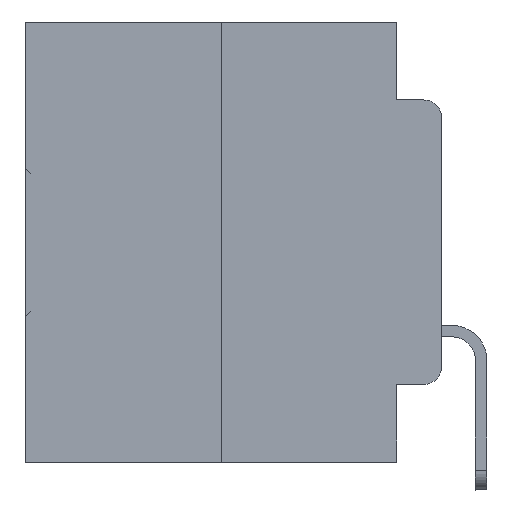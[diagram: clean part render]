
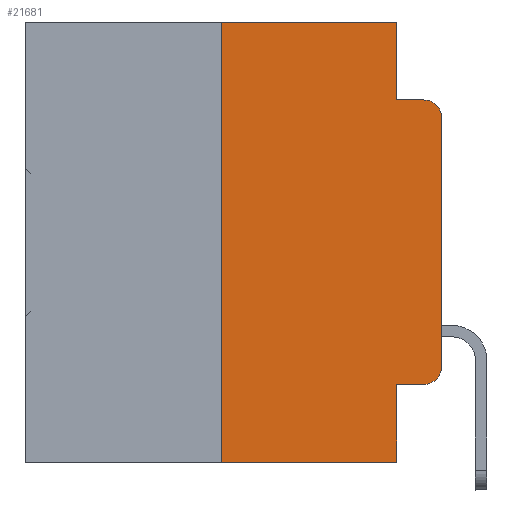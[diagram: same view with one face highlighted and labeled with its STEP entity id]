
A CAD part, left-side view. The second image highlights one B-rep face of the part: STEP entity #21681.
In plain terms, the highlighted planar face has unit normal (-1, 0, 0).
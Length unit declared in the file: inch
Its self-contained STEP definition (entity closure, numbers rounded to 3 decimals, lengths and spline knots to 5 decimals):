
#1292 = ORIENTED_EDGE ( 'NONE', *, *, #23473, .F. ) ;
#1591 = CARTESIAN_POINT ( 'NONE',  ( 0., 0.02, -0.3915 ) ) ;
#1884 = CARTESIAN_POINT ( 'NONE',  ( 0., 0., -0.3915 ) ) ;
#2134 = EDGE_LOOP ( 'NONE', ( #27936, #25136, #20040, #14685, #4754, #1292, #6329, #27400, #12412, #19516 ) ) ;
#2270 = DIRECTION ( 'NONE',  ( -1., 0., 0. ) ) ;
#2576 = VERTEX_POINT ( 'NONE', #7082 ) ;
#3069 = PLANE ( 'NONE',  #4860 ) ;
#3574 = EDGE_CURVE ( 'NONE', #23810, #13026, #19590, .T. ) ;
#4754 = ORIENTED_EDGE ( 'NONE', *, *, #7719, .F. ) ;
#4860 = AXIS2_PLACEMENT_3D ( 'NONE', #28840, #28529, #23282 ) ;
#4862 = AXIS2_PLACEMENT_3D ( 'NONE', #1591, #11908, #27009 ) ;
#5537 = FACE_OUTER_BOUND ( 'NONE', #2134, .T. ) ;
#5858 = CARTESIAN_POINT ( 'NONE',  ( 0., 0.051, -0.4115 ) ) ;
#6103 = CARTESIAN_POINT ( 'NONE',  ( 0., 0., 0. ) ) ;
#6273 = LINE ( 'NONE', #6103, #16764 ) ;
#6329 = ORIENTED_EDGE ( 'NONE', *, *, #15180, .T. ) ;
#6672 = VECTOR ( 'NONE', #7760, 39.37008 ) ;
#7082 = CARTESIAN_POINT ( 'NONE',  ( 0., 0.051, -0.0885 ) ) ;
#7381 = VERTEX_POINT ( 'NONE', #8711 ) ;
#7646 = EDGE_CURVE ( 'NONE', #13026, #32283, #6273, .T. ) ;
#7719 = EDGE_CURVE ( 'NONE', #8173, #29139, #9376, .T. ) ;
#7760 = DIRECTION ( 'NONE',  ( 0., 0., -1. ) ) ;
#7923 = LINE ( 'NONE', #17933, #6672 ) ;
#8173 = VERTEX_POINT ( 'NONE', #12120 ) ;
#8487 = DIRECTION ( 'NONE',  ( 0., -1., 0. ) ) ;
#8711 = CARTESIAN_POINT ( 'NONE',  ( 0., 0.02, -0.0885 ) ) ;
#9376 = LINE ( 'NONE', #19541, #25667 ) ;
#9983 = DIRECTION ( 'NONE',  ( 0., 0., -1. ) ) ;
#10020 = VERTEX_POINT ( 'NONE', #15995 ) ;
#10776 = LINE ( 'NONE', #5858, #12186 ) ;
#11572 = CARTESIAN_POINT ( 'NONE',  ( 0., 0.051, -0.4115 ) ) ;
#11681 = DIRECTION ( 'NONE',  ( 0., -1., 0. ) ) ;
#11908 = DIRECTION ( 'NONE',  ( -1., 0., 0. ) ) ;
#12089 = EDGE_CURVE ( 'NONE', #32283, #7381, #28801, .T. ) ;
#12120 = CARTESIAN_POINT ( 'NONE',  ( 0., 0.25, 0. ) ) ;
#12186 = VECTOR ( 'NONE', #8487, 39.37008 ) ;
#12412 = ORIENTED_EDGE ( 'NONE', *, *, #21705, .T. ) ;
#13026 = VERTEX_POINT ( 'NONE', #1884 ) ;
#13640 = CARTESIAN_POINT ( 'NONE',  ( 0., 0.051, -0.0885 ) ) ;
#14685 = ORIENTED_EDGE ( 'NONE', *, *, #30703, .F. ) ;
#15180 = EDGE_CURVE ( 'NONE', #10020, #29590, #18626, .T. ) ;
#15658 = CARTESIAN_POINT ( 'NONE',  ( 0., 0.02, -0.4115 ) ) ;
#15777 = DIRECTION ( 'NONE',  ( 0., -1., 0. ) ) ;
#15902 = VECTOR ( 'NONE', #15777, 39.37008 ) ;
#15995 = CARTESIAN_POINT ( 'NONE',  ( 0., 0.25, -0.5 ) ) ;
#16051 = VERTEX_POINT ( 'NONE', #11572 ) ;
#16764 = VECTOR ( 'NONE', #26286, 39.37008 ) ;
#16838 = CARTESIAN_POINT ( 'NONE',  ( 0., 0.051, 0. ) ) ;
#17933 = CARTESIAN_POINT ( 'NONE',  ( 0., 0.051, 0. ) ) ;
#18016 = CARTESIAN_POINT ( 'NONE',  ( 0., 0.25, 0. ) ) ;
#18206 = VECTOR ( 'NONE', #28497, 39.37008 ) ;
#18317 = AXIS2_PLACEMENT_3D ( 'NONE', #22624, #2270, #9983 ) ;
#18626 = LINE ( 'NONE', #23579, #18206 ) ;
#19516 = ORIENTED_EDGE ( 'NONE', *, *, #3574, .T. ) ;
#19541 = CARTESIAN_POINT ( 'NONE',  ( 0., 0.473, 0. ) ) ;
#19590 = CIRCLE ( 'NONE', #4862, 0.02 ) ;
#20040 = ORIENTED_EDGE ( 'NONE', *, *, #24246, .F. ) ;
#20434 = LINE ( 'NONE', #25534, #29259 ) ;
#20853 = LINE ( 'NONE', #13640, #15902 ) ;
#21681 = ADVANCED_FACE ( 'NONE', ( #5537 ), #3069, .F. ) ;
#21705 = EDGE_CURVE ( 'NONE', #16051, #23810, #10776, .T. ) ;
#22624 = CARTESIAN_POINT ( 'NONE',  ( 0., 0.02, -0.1085 ) ) ;
#23243 = VECTOR ( 'NONE', #25575, 39.37008 ) ;
#23282 = DIRECTION ( 'NONE',  ( 0., 0., -1. ) ) ;
#23473 = EDGE_CURVE ( 'NONE', #10020, #8173, #25421, .T. ) ;
#23579 = CARTESIAN_POINT ( 'NONE',  ( 0., 0.473, -0.5 ) ) ;
#23810 = VERTEX_POINT ( 'NONE', #15658 ) ;
#24051 = CARTESIAN_POINT ( 'NONE',  ( 0., 0.051, -0.5 ) ) ;
#24246 = EDGE_CURVE ( 'NONE', #2576, #7381, #20853, .T. ) ;
#25136 = ORIENTED_EDGE ( 'NONE', *, *, #12089, .T. ) ;
#25421 = LINE ( 'NONE', #18016, #23243 ) ;
#25534 = CARTESIAN_POINT ( 'NONE',  ( 0., 0.051, 0. ) ) ;
#25575 = DIRECTION ( 'NONE',  ( 0., 0., 1. ) ) ;
#25667 = VECTOR ( 'NONE', #11681, 39.37008 ) ;
#26286 = DIRECTION ( 'NONE',  ( 0., 0., 1. ) ) ;
#27009 = DIRECTION ( 'NONE',  ( 0., 0., -1. ) ) ;
#27400 = ORIENTED_EDGE ( 'NONE', *, *, #29796, .F. ) ;
#27805 = CARTESIAN_POINT ( 'NONE',  ( 0., 0., -0.1085 ) ) ;
#27936 = ORIENTED_EDGE ( 'NONE', *, *, #7646, .T. ) ;
#28494 = DIRECTION ( 'NONE',  ( 0., 0., -1. ) ) ;
#28497 = DIRECTION ( 'NONE',  ( 0., -1., 0. ) ) ;
#28529 = DIRECTION ( 'NONE',  ( 1., 0., 0. ) ) ;
#28801 = CIRCLE ( 'NONE', #18317, 0.02 ) ;
#28840 = CARTESIAN_POINT ( 'NONE',  ( 0., 0.473, 0. ) ) ;
#29139 = VERTEX_POINT ( 'NONE', #16838 ) ;
#29259 = VECTOR ( 'NONE', #28494, 39.37008 ) ;
#29590 = VERTEX_POINT ( 'NONE', #24051 ) ;
#29796 = EDGE_CURVE ( 'NONE', #16051, #29590, #7923, .T. ) ;
#30703 = EDGE_CURVE ( 'NONE', #29139, #2576, #20434, .T. ) ;
#32283 = VERTEX_POINT ( 'NONE', #27805 ) ;
